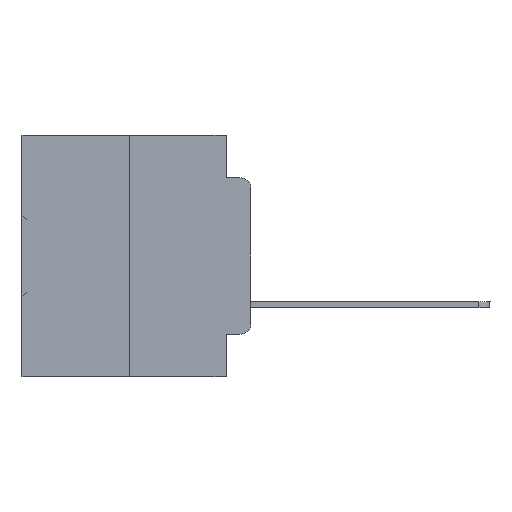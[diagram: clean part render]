
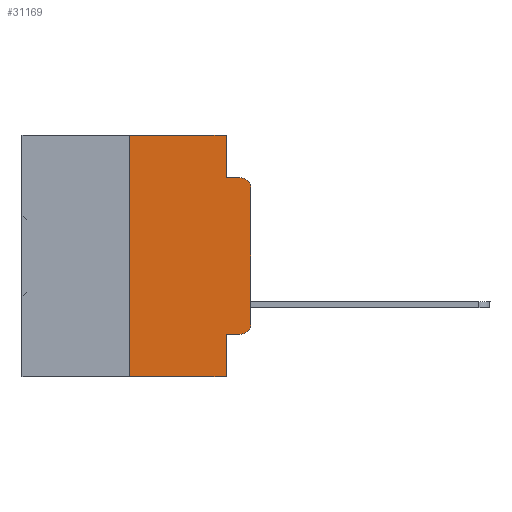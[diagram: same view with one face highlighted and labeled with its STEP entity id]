
A CAD part, left-side view. The second image highlights one B-rep face of the part: STEP entity #31169.
In plain terms, the highlighted planar face has unit normal (-1, 0, 0).
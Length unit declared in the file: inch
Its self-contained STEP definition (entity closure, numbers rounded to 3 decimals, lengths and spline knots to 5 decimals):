
#626 = CARTESIAN_POINT ( 'NONE',  ( 0., 0.25, -0.5 ) ) ;
#849 = VECTOR ( 'NONE', #14752, 39.37008 ) ;
#1091 = CARTESIAN_POINT ( 'NONE',  ( 0., 0., 0. ) ) ;
#3117 = AXIS2_PLACEMENT_3D ( 'NONE', #17983, #20695, #15653 ) ;
#3159 = ORIENTED_EDGE ( 'NONE', *, *, #13793, .T. ) ;
#3202 = ORIENTED_EDGE ( 'NONE', *, *, #36230, .T. ) ;
#3306 = LINE ( 'NONE', #20889, #12454 ) ;
#3764 = CARTESIAN_POINT ( 'NONE',  ( 0., 0.051, 0. ) ) ;
#4322 = CARTESIAN_POINT ( 'NONE',  ( 0., 0.02, -0.4115 ) ) ;
#4875 = CARTESIAN_POINT ( 'NONE',  ( 0., 0.051, 0. ) ) ;
#4876 = VECTOR ( 'NONE', #20659, 39.37008 ) ;
#6287 = ORIENTED_EDGE ( 'NONE', *, *, #32683, .F. ) ;
#6476 = CARTESIAN_POINT ( 'NONE',  ( 0., 0.473, -0.5 ) ) ;
#6810 = VERTEX_POINT ( 'NONE', #22101 ) ;
#6849 = VERTEX_POINT ( 'NONE', #21863 ) ;
#7300 = VERTEX_POINT ( 'NONE', #4322 ) ;
#7967 = EDGE_CURVE ( 'NONE', #9448, #6849, #11366, .T. ) ;
#8696 = ORIENTED_EDGE ( 'NONE', *, *, #8805, .F. ) ;
#8805 = EDGE_CURVE ( 'NONE', #34664, #6849, #35927, .T. ) ;
#9448 = VERTEX_POINT ( 'NONE', #626 ) ;
#10095 = CARTESIAN_POINT ( 'NONE',  ( 0., 0.02, -0.1085 ) ) ;
#10419 = CARTESIAN_POINT ( 'NONE',  ( 0., 0.051, 0. ) ) ;
#11366 = LINE ( 'NONE', #6476, #849 ) ;
#11836 = CIRCLE ( 'NONE', #32729, 0.02 ) ;
#11978 = DIRECTION ( 'NONE',  ( 0., 0., 1. ) ) ;
#12361 = ORIENTED_EDGE ( 'NONE', *, *, #7967, .T. ) ;
#12449 = DIRECTION ( 'NONE',  ( 0., 0., -1. ) ) ;
#12454 = VECTOR ( 'NONE', #11978, 39.37008 ) ;
#12556 = VERTEX_POINT ( 'NONE', #27163 ) ;
#12655 = DIRECTION ( 'NONE',  ( 0., 0., -1. ) ) ;
#13793 = EDGE_CURVE ( 'NONE', #12556, #6810, #11836, .T. ) ;
#14728 = ORIENTED_EDGE ( 'NONE', *, *, #24937, .F. ) ;
#14752 = DIRECTION ( 'NONE',  ( 0., -1., 0. ) ) ;
#14821 = EDGE_CURVE ( 'NONE', #9448, #20981, #3306, .T. ) ;
#15653 = DIRECTION ( 'NONE',  ( 0., 0., -1. ) ) ;
#15922 = CARTESIAN_POINT ( 'NONE',  ( 0., 0.25, 0. ) ) ;
#16239 = DIRECTION ( 'NONE',  ( 1., 0., 0. ) ) ;
#16515 = VECTOR ( 'NONE', #32709, 39.37008 ) ;
#17402 = VERTEX_POINT ( 'NONE', #10419 ) ;
#17983 = CARTESIAN_POINT ( 'NONE',  ( 0., 0.02, -0.3915 ) ) ;
#19069 = CARTESIAN_POINT ( 'NONE',  ( 0., 0.473, 0. ) ) ;
#20350 = LINE ( 'NONE', #23263, #26097 ) ;
#20659 = DIRECTION ( 'NONE',  ( 0., 0., 1. ) ) ;
#20695 = DIRECTION ( 'NONE',  ( -1., 0., 0. ) ) ;
#20800 = DIRECTION ( 'NONE',  ( 0., -1., 0. ) ) ;
#20889 = CARTESIAN_POINT ( 'NONE',  ( 0., 0.25, 0. ) ) ;
#20981 = VERTEX_POINT ( 'NONE', #15922 ) ;
#21204 = DIRECTION ( 'NONE',  ( -1., 0., 0. ) ) ;
#21863 = CARTESIAN_POINT ( 'NONE',  ( 0., 0.051, -0.5 ) ) ;
#22101 = CARTESIAN_POINT ( 'NONE',  ( 0., 0.02, -0.0885 ) ) ;
#22156 = EDGE_CURVE ( 'NONE', #26771, #12556, #35635, .T. ) ;
#23263 = CARTESIAN_POINT ( 'NONE',  ( 0., 0.051, -0.4115 ) ) ;
#23716 = CIRCLE ( 'NONE', #3117, 0.02 ) ;
#23749 = CARTESIAN_POINT ( 'NONE',  ( 0., 0., -0.3915 ) ) ;
#24044 = EDGE_CURVE ( 'NONE', #7300, #26771, #23716, .T. ) ;
#24120 = AXIS2_PLACEMENT_3D ( 'NONE', #19069, #16239, #24753 ) ;
#24542 = CARTESIAN_POINT ( 'NONE',  ( 0., 0.473, 0. ) ) ;
#24753 = DIRECTION ( 'NONE',  ( 0., 0., -1. ) ) ;
#24937 = EDGE_CURVE ( 'NONE', #35077, #6810, #35606, .T. ) ;
#26097 = VECTOR ( 'NONE', #20800, 39.37008 ) ;
#26651 = VECTOR ( 'NONE', #27460, 39.37008 ) ;
#26771 = VERTEX_POINT ( 'NONE', #23749 ) ;
#27135 = CARTESIAN_POINT ( 'NONE',  ( 0., 0.051, -0.0885 ) ) ;
#27163 = CARTESIAN_POINT ( 'NONE',  ( 0., 0., -0.1085 ) ) ;
#27460 = DIRECTION ( 'NONE',  ( 0., 0., -1. ) ) ;
#28674 = EDGE_CURVE ( 'NONE', #20981, #17402, #31534, .T. ) ;
#28735 = ORIENTED_EDGE ( 'NONE', *, *, #14821, .F. ) ;
#30073 = DIRECTION ( 'NONE',  ( 0., -1., 0. ) ) ;
#30151 = FACE_OUTER_BOUND ( 'NONE', #35725, .T. ) ;
#31169 = ADVANCED_FACE ( 'NONE', ( #30151 ), #36208, .F. ) ;
#31252 = ORIENTED_EDGE ( 'NONE', *, *, #24044, .T. ) ;
#31534 = LINE ( 'NONE', #24542, #16515 ) ;
#31770 = LINE ( 'NONE', #3764, #36176 ) ;
#32683 = EDGE_CURVE ( 'NONE', #17402, #35077, #31770, .T. ) ;
#32709 = DIRECTION ( 'NONE',  ( 0., -1., 0. ) ) ;
#32729 = AXIS2_PLACEMENT_3D ( 'NONE', #10095, #21204, #12655 ) ;
#33152 = CARTESIAN_POINT ( 'NONE',  ( 0., 0.051, -0.0885 ) ) ;
#33771 = ORIENTED_EDGE ( 'NONE', *, *, #22156, .T. ) ;
#34664 = VERTEX_POINT ( 'NONE', #36150 ) ;
#34706 = VECTOR ( 'NONE', #30073, 39.37008 ) ;
#35077 = VERTEX_POINT ( 'NONE', #27135 ) ;
#35336 = ORIENTED_EDGE ( 'NONE', *, *, #28674, .F. ) ;
#35606 = LINE ( 'NONE', #33152, #34706 ) ;
#35635 = LINE ( 'NONE', #1091, #4876 ) ;
#35725 = EDGE_LOOP ( 'NONE', ( #33771, #3159, #14728, #6287, #35336, #28735, #12361, #8696, #3202, #31252 ) ) ;
#35927 = LINE ( 'NONE', #4875, #26651 ) ;
#36150 = CARTESIAN_POINT ( 'NONE',  ( 0., 0.051, -0.4115 ) ) ;
#36176 = VECTOR ( 'NONE', #12449, 39.37008 ) ;
#36208 = PLANE ( 'NONE',  #24120 ) ;
#36230 = EDGE_CURVE ( 'NONE', #34664, #7300, #20350, .T. ) ;
